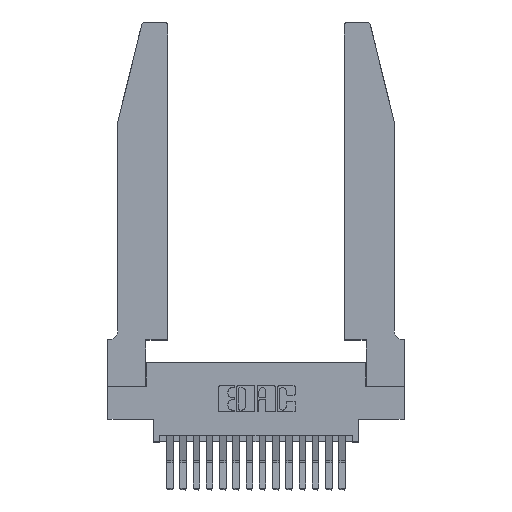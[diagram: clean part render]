
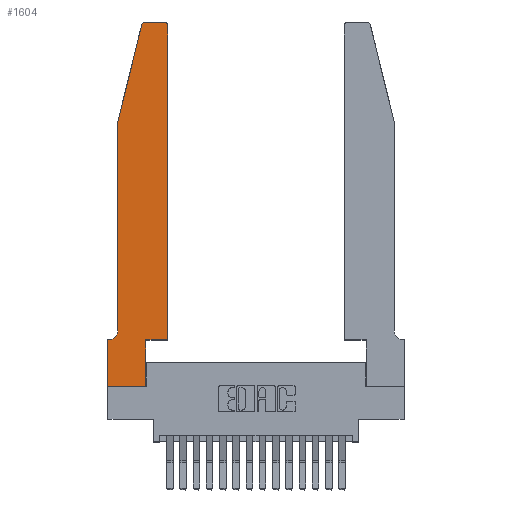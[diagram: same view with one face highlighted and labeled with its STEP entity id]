
A CAD part, top view. The second image highlights one B-rep face of the part: STEP entity #1604.
In plain terms, the highlighted planar face has unit normal (0, 0, 1).
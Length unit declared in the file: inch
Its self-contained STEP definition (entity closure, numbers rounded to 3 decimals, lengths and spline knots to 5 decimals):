
#131 = VERTEX_POINT ( 'NONE', #14482 ) ;
#229 = EDGE_CURVE ( 'NONE', #9918, #13981, #14239, .T. ) ;
#509 = EDGE_CURVE ( 'NONE', #5470, #131, #13540, .T. ) ;
#1082 = VERTEX_POINT ( 'NONE', #12108 ) ;
#1158 = LINE ( 'NONE', #15232, #12993 ) ;
#1484 = CARTESIAN_POINT ( 'NONE',  ( 0., 0.35, 0.37 ) ) ;
#1604 = ADVANCED_FACE ( 'NONE', ( #15500 ), #5515, .T. ) ;
#1608 = DIRECTION ( 'NONE',  ( 0., 0., 1. ) ) ;
#2134 = AXIS2_PLACEMENT_3D ( 'NONE', #13397, #4232, #14874 ) ;
#2207 = VECTOR ( 'NONE', #8397, 39.37008 ) ;
#2282 = ORIENTED_EDGE ( 'NONE', *, *, #18985, .T. ) ;
#2362 = LINE ( 'NONE', #11909, #10116 ) ;
#2547 = DIRECTION ( 'NONE',  ( -0.239, -0.971, 0. ) ) ;
#2550 = VECTOR ( 'NONE', #5208, 39.37008 ) ;
#2770 = LINE ( 'NONE', #10213, #18433 ) ;
#2867 = LINE ( 'NONE', #13362, #10596 ) ;
#3052 = LINE ( 'NONE', #9753, #2550 ) ;
#3170 = EDGE_CURVE ( 'NONE', #15284, #9918, #2770, .T. ) ;
#3655 = ORIENTED_EDGE ( 'NONE', *, *, #509, .T. ) ;
#3803 = DIRECTION ( 'NONE',  ( 1., 0., 0. ) ) ;
#3843 = DIRECTION ( 'NONE',  ( 0., 0., 1. ) ) ;
#4219 = CARTESIAN_POINT ( 'NONE',  ( 0.0755, 2., 0.37 ) ) ;
#4232 = DIRECTION ( 'NONE',  ( 0., 0., -1. ) ) ;
#4604 = DIRECTION ( 'NONE',  ( -1., 0., 0. ) ) ;
#4627 = ORIENTED_EDGE ( 'NONE', *, *, #12362, .T. ) ;
#5208 = DIRECTION ( 'NONE',  ( 0., 1., 0. ) ) ;
#5243 = LINE ( 'NONE', #9792, #9299 ) ;
#5338 = CARTESIAN_POINT ( 'NONE',  ( 0.25487, 2.72718, 0.37 ) ) ;
#5422 = VECTOR ( 'NONE', #18706, 39.37008 ) ;
#5470 = VERTEX_POINT ( 'NONE', #9921 ) ;
#5515 = PLANE ( 'NONE',  #16009 ) ;
#5555 = CARTESIAN_POINT ( 'NONE',  ( 0., 0.35, 0.37 ) ) ;
#5660 = EDGE_CURVE ( 'NONE', #13981, #1082, #6337, .T. ) ;
#5752 = DIRECTION ( 'NONE',  ( 0., 1., 0. ) ) ;
#5771 = AXIS2_PLACEMENT_3D ( 'NONE', #10873, #1608, #12422 ) ;
#6337 = LINE ( 'NONE', #4219, #13965 ) ;
#8018 = ORIENTED_EDGE ( 'NONE', *, *, #229, .T. ) ;
#8117 = ORIENTED_EDGE ( 'NONE', *, *, #14445, .T. ) ;
#8397 = DIRECTION ( 'NONE',  ( 0., -1., 0. ) ) ;
#8975 = CARTESIAN_POINT ( 'NONE',  ( 0.0055, 0.35, 0.37 ) ) ;
#9299 = VECTOR ( 'NONE', #17268, 39.37008 ) ;
#9499 = EDGE_CURVE ( 'NONE', #9818, #12046, #14447, .T. ) ;
#9690 = ORIENTED_EDGE ( 'NONE', *, *, #12322, .T. ) ;
#9691 = ORIENTED_EDGE ( 'NONE', *, *, #3170, .T. ) ;
#9753 = CARTESIAN_POINT ( 'NONE',  ( 0.2865, 0.35, 0.37 ) ) ;
#9792 = CARTESIAN_POINT ( 'NONE',  ( 0.0755, 2., 0.37 ) ) ;
#9818 = VERTEX_POINT ( 'NONE', #1484 ) ;
#9918 = VERTEX_POINT ( 'NONE', #12430 ) ;
#9921 = CARTESIAN_POINT ( 'NONE',  ( 0.2865, 0.35, 0.37 ) ) ;
#9949 = CIRCLE ( 'NONE', #5771, 0.03 ) ;
#10116 = VECTOR ( 'NONE', #10364, 39.37008 ) ;
#10213 = CARTESIAN_POINT ( 'NONE',  ( 0.2605, 2.75, 0.37 ) ) ;
#10338 = CARTESIAN_POINT ( 'NONE',  ( 0.2865, 0., 0.37 ) ) ;
#10364 = DIRECTION ( 'NONE',  ( 1., 0., 0. ) ) ;
#10596 = VECTOR ( 'NONE', #5752, 39.37008 ) ;
#10723 = CARTESIAN_POINT ( 'NONE',  ( 0.284, 2.72, 0.37 ) ) ;
#10873 = CARTESIAN_POINT ( 'NONE',  ( 0.4205, 2.72, 0.37 ) ) ;
#11012 = CARTESIAN_POINT ( 'NONE',  ( 0.0755, 0.42, 0.37 ) ) ;
#11807 = DIRECTION ( 'NONE',  ( -1., 0., 0. ) ) ;
#11909 = CARTESIAN_POINT ( 'NONE',  ( 0., 0., 0.37 ) ) ;
#12046 = VERTEX_POINT ( 'NONE', #12798 ) ;
#12108 = CARTESIAN_POINT ( 'NONE',  ( 0.0755, 2., 0.37 ) ) ;
#12322 = EDGE_CURVE ( 'NONE', #131, #17086, #2867, .T. ) ;
#12362 = EDGE_CURVE ( 'NONE', #12046, #18981, #2362, .T. ) ;
#12422 = DIRECTION ( 'NONE',  ( 1., 0., 0. ) ) ;
#12430 = CARTESIAN_POINT ( 'NONE',  ( 0.284, 2.75, 0.37 ) ) ;
#12597 = ORIENTED_EDGE ( 'NONE', *, *, #5660, .T. ) ;
#12798 = CARTESIAN_POINT ( 'NONE',  ( 0., 0., 0.37 ) ) ;
#12993 = VECTOR ( 'NONE', #4604, 39.37008 ) ;
#13362 = CARTESIAN_POINT ( 'NONE',  ( 0.4505, 0.35, 0.37 ) ) ;
#13397 = CARTESIAN_POINT ( 'NONE',  ( 0.0055, 0.42, 0.37 ) ) ;
#13493 = ORIENTED_EDGE ( 'NONE', *, *, #13948, .T. ) ;
#13540 = LINE ( 'NONE', #16363, #5422 ) ;
#13948 = EDGE_CURVE ( 'NONE', #18981, #5470, #3052, .T. ) ;
#13965 = VECTOR ( 'NONE', #2547, 39.37008 ) ;
#13981 = VERTEX_POINT ( 'NONE', #5338 ) ;
#14239 = CIRCLE ( 'NONE', #17475, 0.03 ) ;
#14445 = EDGE_CURVE ( 'NONE', #1082, #19230, #5243, .T. ) ;
#14447 = LINE ( 'NONE', #17342, #2207 ) ;
#14482 = CARTESIAN_POINT ( 'NONE',  ( 0.4505, 0.35, 0.37 ) ) ;
#14807 = VERTEX_POINT ( 'NONE', #8975 ) ;
#14874 = DIRECTION ( 'NONE',  ( -1., 0., 0. ) ) ;
#15232 = CARTESIAN_POINT ( 'NONE',  ( 0.0755, 0.35, 0.37 ) ) ;
#15284 = VERTEX_POINT ( 'NONE', #16406 ) ;
#15500 = FACE_OUTER_BOUND ( 'NONE', #16476, .T. ) ;
#16009 = AXIS2_PLACEMENT_3D ( 'NONE', #5555, #3843, #3803 ) ;
#16039 = EDGE_CURVE ( 'NONE', #17086, #15284, #9949, .T. ) ;
#16050 = ORIENTED_EDGE ( 'NONE', *, *, #16039, .T. ) ;
#16363 = CARTESIAN_POINT ( 'NONE',  ( 0.4505, 0.35, 0.37 ) ) ;
#16406 = CARTESIAN_POINT ( 'NONE',  ( 0.4205, 2.75, 0.37 ) ) ;
#16476 = EDGE_LOOP ( 'NONE', ( #9691, #8018, #12597, #8117, #2282, #16847, #17578, #4627, #13493, #3655, #9690, #16050 ) ) ;
#16847 = ORIENTED_EDGE ( 'NONE', *, *, #18623, .T. ) ;
#17086 = VERTEX_POINT ( 'NONE', #19148 ) ;
#17207 = DIRECTION ( 'NONE',  ( 1., 0., 0. ) ) ;
#17268 = DIRECTION ( 'NONE',  ( 0., -1., 0. ) ) ;
#17342 = CARTESIAN_POINT ( 'NONE',  ( 0., 0., 0.37 ) ) ;
#17475 = AXIS2_PLACEMENT_3D ( 'NONE', #10723, #17605, #17207 ) ;
#17578 = ORIENTED_EDGE ( 'NONE', *, *, #9499, .T. ) ;
#17605 = DIRECTION ( 'NONE',  ( 0., 0., 1. ) ) ;
#18433 = VECTOR ( 'NONE', #11807, 39.37008 ) ;
#18623 = EDGE_CURVE ( 'NONE', #14807, #9818, #1158, .T. ) ;
#18706 = DIRECTION ( 'NONE',  ( 1., 0., 0. ) ) ;
#18981 = VERTEX_POINT ( 'NONE', #10338 ) ;
#18985 = EDGE_CURVE ( 'NONE', #19230, #14807, #19203, .T. ) ;
#19148 = CARTESIAN_POINT ( 'NONE',  ( 0.4505, 2.72, 0.37 ) ) ;
#19203 = CIRCLE ( 'NONE', #2134, 0.07 ) ;
#19230 = VERTEX_POINT ( 'NONE', #11012 ) ;
